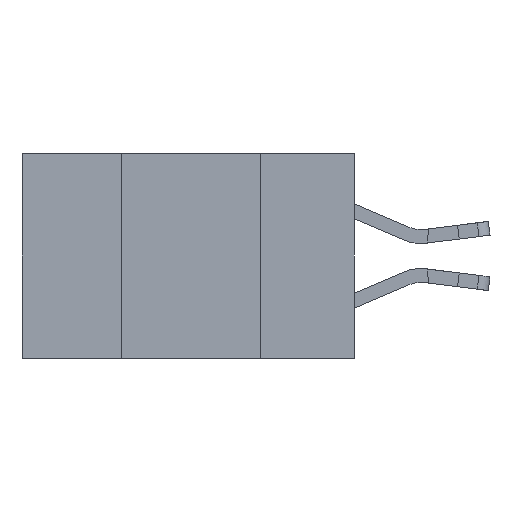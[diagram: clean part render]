
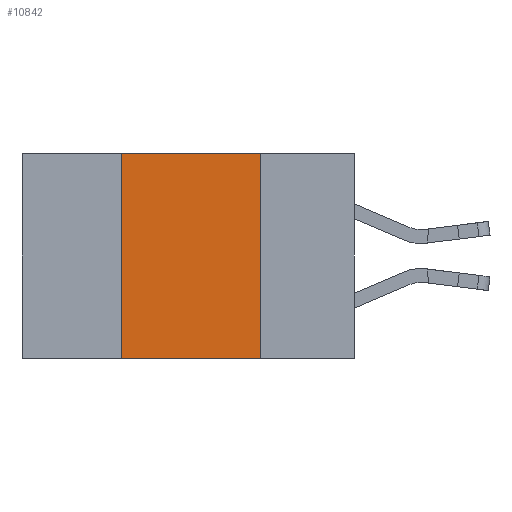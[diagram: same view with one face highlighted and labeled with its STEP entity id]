
A CAD part, left-side view. The second image highlights one B-rep face of the part: STEP entity #10842.
In plain terms, the highlighted planar face has unit normal (-1, 0, 0).
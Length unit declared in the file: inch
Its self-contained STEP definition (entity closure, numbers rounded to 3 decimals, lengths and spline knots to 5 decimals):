
#351 = DIRECTION ( 'NONE',  ( 0., 0., -1. ) ) ;
#836 = EDGE_CURVE ( 'NONE', #2396, #4295, #5767, .T. ) ;
#937 = DIRECTION ( 'NONE',  ( 1., 0., 0. ) ) ;
#2047 = PLANE ( 'NONE',  #5934 ) ;
#2396 = VERTEX_POINT ( 'NONE', #2714 ) ;
#2496 = EDGE_CURVE ( 'NONE', #2396, #2620, #11106, .T. ) ;
#2620 = VERTEX_POINT ( 'NONE', #11832 ) ;
#2714 = CARTESIAN_POINT ( 'NONE',  ( 0., 0.42, -0.37 ) ) ;
#3133 = EDGE_CURVE ( 'NONE', #2620, #9965, #3135, .T. ) ;
#3135 = LINE ( 'NONE', #4253, #7531 ) ;
#3871 = EDGE_LOOP ( 'NONE', ( #4106, #6732, #12692, #15800 ) ) ;
#4106 = ORIENTED_EDGE ( 'NONE', *, *, #12033, .F. ) ;
#4210 = VECTOR ( 'NONE', #13585, 39.37008 ) ;
#4253 = CARTESIAN_POINT ( 'NONE',  ( 0., 0.6, 0. ) ) ;
#4295 = VERTEX_POINT ( 'NONE', #13572 ) ;
#4860 = VECTOR ( 'NONE', #351, 39.37008 ) ;
#5767 = LINE ( 'NONE', #9703, #9023 ) ;
#5934 = AXIS2_PLACEMENT_3D ( 'NONE', #12636, #937, #6146 ) ;
#6146 = DIRECTION ( 'NONE',  ( 0., 0., -1. ) ) ;
#6732 = ORIENTED_EDGE ( 'NONE', *, *, #3133, .F. ) ;
#7355 = FACE_OUTER_BOUND ( 'NONE', #3871, .T. ) ;
#7531 = VECTOR ( 'NONE', #10857, 39.37008 ) ;
#8362 = CARTESIAN_POINT ( 'NONE',  ( 0., 0.42, -0.37 ) ) ;
#9023 = VECTOR ( 'NONE', #12343, 39.37008 ) ;
#9703 = CARTESIAN_POINT ( 'NONE',  ( 0., 0.6, -0.37 ) ) ;
#9837 = LINE ( 'NONE', #12058, #4860 ) ;
#9965 = VERTEX_POINT ( 'NONE', #12447 ) ;
#10842 = ADVANCED_FACE ( 'NONE', ( #7355 ), #2047, .F. ) ;
#10857 = DIRECTION ( 'NONE',  ( 0., -1., 0. ) ) ;
#11106 = LINE ( 'NONE', #8362, #4210 ) ;
#11832 = CARTESIAN_POINT ( 'NONE',  ( 0., 0.42, 0. ) ) ;
#12033 = EDGE_CURVE ( 'NONE', #9965, #4295, #9837, .T. ) ;
#12058 = CARTESIAN_POINT ( 'NONE',  ( 0., 0.17, -0.37 ) ) ;
#12343 = DIRECTION ( 'NONE',  ( 0., -1., 0. ) ) ;
#12447 = CARTESIAN_POINT ( 'NONE',  ( 0., 0.17, 0. ) ) ;
#12636 = CARTESIAN_POINT ( 'NONE',  ( 0., 0.6, 0. ) ) ;
#12692 = ORIENTED_EDGE ( 'NONE', *, *, #2496, .F. ) ;
#13572 = CARTESIAN_POINT ( 'NONE',  ( 0., 0.17, -0.37 ) ) ;
#13585 = DIRECTION ( 'NONE',  ( 0., 0., 1. ) ) ;
#15800 = ORIENTED_EDGE ( 'NONE', *, *, #836, .T. ) ;
